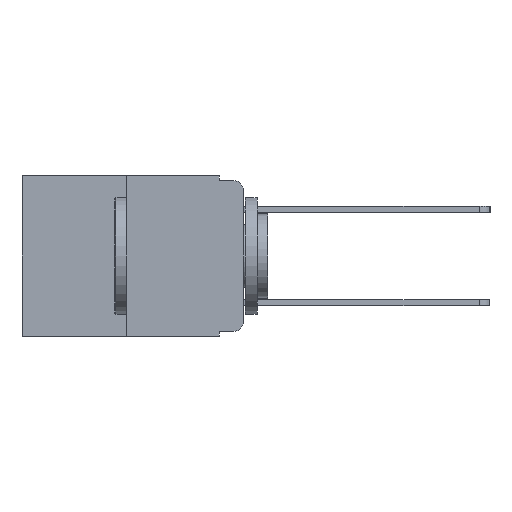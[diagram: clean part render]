
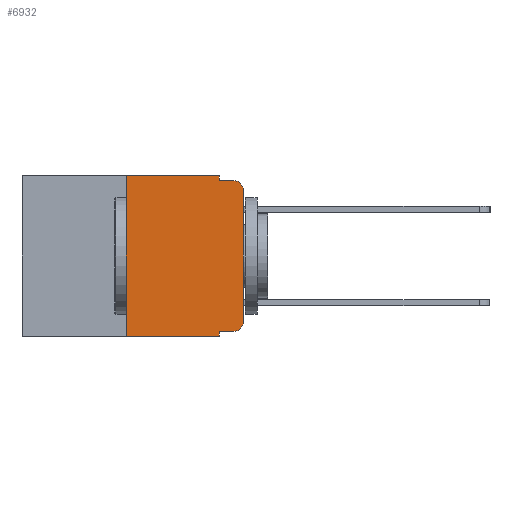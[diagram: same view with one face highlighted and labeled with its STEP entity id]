
A CAD part, left-side view. The second image highlights one B-rep face of the part: STEP entity #6932.
In plain terms, the highlighted planar face has unit normal (-1, 0, 0).
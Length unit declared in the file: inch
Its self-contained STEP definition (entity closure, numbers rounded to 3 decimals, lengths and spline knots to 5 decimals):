
#199 = ORIENTED_EDGE ( 'NONE', *, *, #3688, .F. ) ;
#205 = LINE ( 'NONE', #4183, #2500 ) ;
#258 = DIRECTION ( 'NONE',  ( 0., 0., 1. ) ) ;
#806 = ORIENTED_EDGE ( 'NONE', *, *, #9369, .F. ) ;
#844 = DIRECTION ( 'NONE',  ( 0., -1., 0. ) ) ;
#960 = CIRCLE ( 'NONE', #2202, 0.02 ) ;
#966 = ORIENTED_EDGE ( 'NONE', *, *, #11537, .T. ) ;
#1073 = CARTESIAN_POINT ( 'NONE',  ( 0., 0., -0.313 ) ) ;
#1297 = LINE ( 'NONE', #6867, #6264 ) ;
#1681 = FACE_OUTER_BOUND ( 'NONE', #8617, .T. ) ;
#2202 = AXIS2_PLACEMENT_3D ( 'NONE', #10360, #4780, #11230 ) ;
#2234 = VECTOR ( 'NONE', #844, 39.37008 ) ;
#2339 = VECTOR ( 'NONE', #8787, 39.37008 ) ;
#2476 = VERTEX_POINT ( 'NONE', #7378 ) ;
#2500 = VECTOR ( 'NONE', #258, 39.37008 ) ;
#2593 = VERTEX_POINT ( 'NONE', #7612 ) ;
#2912 = AXIS2_PLACEMENT_3D ( 'NONE', #11334, #5875, #12185 ) ;
#3214 = DIRECTION ( 'NONE',  ( 0., -1., 0. ) ) ;
#3224 = CARTESIAN_POINT ( 'NONE',  ( 0., 0.051, 0. ) ) ;
#3479 = VECTOR ( 'NONE', #10500, 39.37008 ) ;
#3540 = CARTESIAN_POINT ( 'NONE',  ( 0., 0.25, 0. ) ) ;
#3594 = AXIS2_PLACEMENT_3D ( 'NONE', #9644, #3990, #10530 ) ;
#3688 = EDGE_CURVE ( 'NONE', #8163, #11783, #10401, .T. ) ;
#3763 = EDGE_CURVE ( 'NONE', #2593, #9977, #1297, .T. ) ;
#3809 = VERTEX_POINT ( 'NONE', #1073 ) ;
#3948 = CARTESIAN_POINT ( 'NONE',  ( 0., 0.473, 0. ) ) ;
#3990 = DIRECTION ( 'NONE',  ( -1., 0., 0. ) ) ;
#4024 = CIRCLE ( 'NONE', #3594, 0.02 ) ;
#4045 = LINE ( 'NONE', #9789, #9128 ) ;
#4183 = CARTESIAN_POINT ( 'NONE',  ( 0., 0., 0. ) ) ;
#4223 = CARTESIAN_POINT ( 'NONE',  ( 0., 0.051, 0. ) ) ;
#4269 = DIRECTION ( 'NONE',  ( 0., 0., -1. ) ) ;
#4780 = DIRECTION ( 'NONE',  ( -1., 0., 0. ) ) ;
#5150 = ORIENTED_EDGE ( 'NONE', *, *, #11614, .F. ) ;
#5429 = VECTOR ( 'NONE', #8994, 39.37008 ) ;
#5440 = VERTEX_POINT ( 'NONE', #7834 ) ;
#5764 = VERTEX_POINT ( 'NONE', #8441 ) ;
#5875 = DIRECTION ( 'NONE',  ( 1., 0., 0. ) ) ;
#6204 = CARTESIAN_POINT ( 'NONE',  ( 0., 0.051, 0. ) ) ;
#6264 = VECTOR ( 'NONE', #3214, 39.37008 ) ;
#6709 = CARTESIAN_POINT ( 'NONE',  ( 0., 0.051, -0.01 ) ) ;
#6867 = CARTESIAN_POINT ( 'NONE',  ( 0., 0.051, -0.333 ) ) ;
#6932 = ADVANCED_FACE ( 'NONE', ( #1681 ), #8691, .F. ) ;
#6946 = ORIENTED_EDGE ( 'NONE', *, *, #11134, .T. ) ;
#6967 = EDGE_CURVE ( 'NONE', #9977, #3809, #4024, .T. ) ;
#7367 = CARTESIAN_POINT ( 'NONE',  ( 0., 0.051, -0.01 ) ) ;
#7378 = CARTESIAN_POINT ( 'NONE',  ( 0., 0., -0.03 ) ) ;
#7601 = EDGE_CURVE ( 'NONE', #2593, #5440, #10165, .T. ) ;
#7612 = CARTESIAN_POINT ( 'NONE',  ( 0., 0.051, -0.333 ) ) ;
#7792 = VECTOR ( 'NONE', #4269, 39.37008 ) ;
#7834 = CARTESIAN_POINT ( 'NONE',  ( 0., 0.051, -0.343 ) ) ;
#8143 = LINE ( 'NONE', #10513, #2339 ) ;
#8163 = VERTEX_POINT ( 'NONE', #7367 ) ;
#8441 = CARTESIAN_POINT ( 'NONE',  ( 0., 0.25, -0.343 ) ) ;
#8580 = ORIENTED_EDGE ( 'NONE', *, *, #7601, .F. ) ;
#8617 = EDGE_LOOP ( 'NONE', ( #6946, #11832, #199, #5150, #806, #11465, #966, #8580, #11477, #9974 ) ) ;
#8691 = PLANE ( 'NONE',  #2912 ) ;
#8787 = DIRECTION ( 'NONE',  ( 0., 0., 1. ) ) ;
#8994 = DIRECTION ( 'NONE',  ( 0., 0., -1. ) ) ;
#9128 = VECTOR ( 'NONE', #9745, 39.37008 ) ;
#9369 = EDGE_CURVE ( 'NONE', #10599, #9607, #11210, .T. ) ;
#9607 = VERTEX_POINT ( 'NONE', #6204 ) ;
#9644 = CARTESIAN_POINT ( 'NONE',  ( 0., 0.02, -0.313 ) ) ;
#9745 = DIRECTION ( 'NONE',  ( 0., -1., 0. ) ) ;
#9789 = CARTESIAN_POINT ( 'NONE',  ( 0., 0.473, -0.343 ) ) ;
#9974 = ORIENTED_EDGE ( 'NONE', *, *, #6967, .T. ) ;
#9977 = VERTEX_POINT ( 'NONE', #10339 ) ;
#10165 = LINE ( 'NONE', #3224, #7792 ) ;
#10339 = CARTESIAN_POINT ( 'NONE',  ( 0., 0.02, -0.333 ) ) ;
#10347 = LINE ( 'NONE', #4223, #5429 ) ;
#10360 = CARTESIAN_POINT ( 'NONE',  ( 0., 0.02, -0.03 ) ) ;
#10401 = LINE ( 'NONE', #6709, #2234 ) ;
#10500 = DIRECTION ( 'NONE',  ( 0., -1., 0. ) ) ;
#10513 = CARTESIAN_POINT ( 'NONE',  ( 0., 0.25, 0. ) ) ;
#10530 = DIRECTION ( 'NONE',  ( 0., 0., -1. ) ) ;
#10599 = VERTEX_POINT ( 'NONE', #3540 ) ;
#10780 = EDGE_CURVE ( 'NONE', #2476, #11783, #960, .T. ) ;
#11134 = EDGE_CURVE ( 'NONE', #3809, #2476, #205, .T. ) ;
#11210 = LINE ( 'NONE', #3948, #3479 ) ;
#11230 = DIRECTION ( 'NONE',  ( 0., 0., -1. ) ) ;
#11334 = CARTESIAN_POINT ( 'NONE',  ( 0., 0.473, 0. ) ) ;
#11404 = EDGE_CURVE ( 'NONE', #5764, #10599, #8143, .T. ) ;
#11465 = ORIENTED_EDGE ( 'NONE', *, *, #11404, .F. ) ;
#11477 = ORIENTED_EDGE ( 'NONE', *, *, #3763, .T. ) ;
#11537 = EDGE_CURVE ( 'NONE', #5764, #5440, #4045, .T. ) ;
#11614 = EDGE_CURVE ( 'NONE', #9607, #8163, #10347, .T. ) ;
#11743 = CARTESIAN_POINT ( 'NONE',  ( 0., 0.02, -0.01 ) ) ;
#11783 = VERTEX_POINT ( 'NONE', #11743 ) ;
#11832 = ORIENTED_EDGE ( 'NONE', *, *, #10780, .T. ) ;
#12185 = DIRECTION ( 'NONE',  ( 0., 0., -1. ) ) ;
